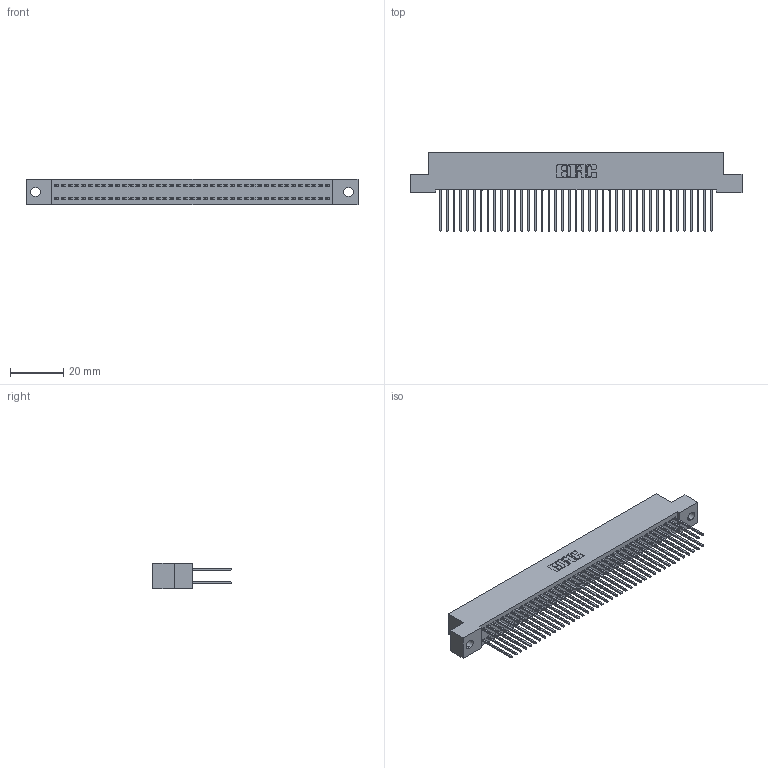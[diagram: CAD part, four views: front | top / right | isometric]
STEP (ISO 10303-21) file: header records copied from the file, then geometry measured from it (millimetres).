
FILE_DESCRIPTION (( 'STEP AP203' ), '1' );
FILE_NAME ('342-082-540-202.STEP', '2019-10-04T12:07:10', ( '' ), ( '' ), 'SwSTEP 2.0', 'SolidWorks 2016', '' );
FILE_SCHEMA (( 'CONFIG_CONTROL_DESIGN' ));
Length unit declared in the file: inch
Products named in the file (3): 342 Part_.128 Slot; 345-292-001_345-293-140; 342-082-540-202
Assembly tree (83 placements, depth 2):
  342-082-540-202
    342 Part_.128 Slot
    345-292-001_345-293-140  x82
Bounding box: 124.46 x 29.47 x 9.4 mm (x, y, z)
Volume: 11436.7 mm3; surface area: 19732.9 mm2
Topology: 83 solids, 83 shells, 4378 faces, 13021 edges, 8570 vertices
Faces by surface type: plane 3022, cylinder 1356
Entity records: 26527 total; most frequent: CARTESIAN_POINT 4398, ORIENTED_EDGE 4334, DIRECTION 3759, EDGE_CURVE 2167, VECTOR 2039, LINE 2039, VERTEX_POINT 1442, AXIS2_PLACEMENT_3D 860
